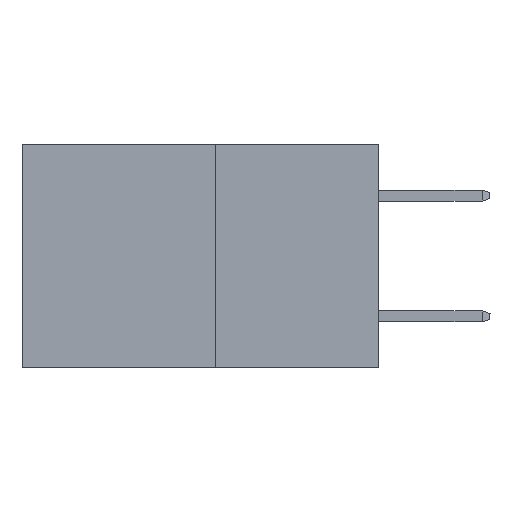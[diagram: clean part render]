
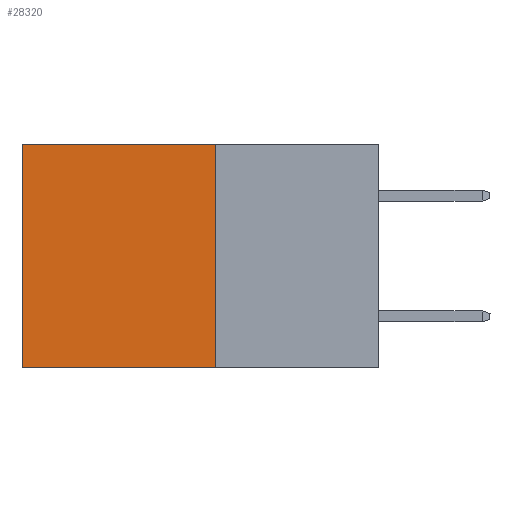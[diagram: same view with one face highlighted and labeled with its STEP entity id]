
A CAD part, left-side view. The second image highlights one B-rep face of the part: STEP entity #28320.
In plain terms, the highlighted planar face has unit normal (-1, 0, 0).
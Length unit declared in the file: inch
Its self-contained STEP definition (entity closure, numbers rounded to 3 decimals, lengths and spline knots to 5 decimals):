
#2869 = EDGE_CURVE ( 'NONE', #17313, #3148, #24031, .T. ) ;
#2882 = CARTESIAN_POINT ( 'NONE',  ( 0.277, 0.59, -0.37 ) ) ;
#3148 = VERTEX_POINT ( 'NONE', #2882 ) ;
#4217 = CARTESIAN_POINT ( 'NONE',  ( 0.277, 0.27, -0.37 ) ) ;
#5641 = ORIENTED_EDGE ( 'NONE', *, *, #2869, .T. ) ;
#6973 = DIRECTION ( 'NONE',  ( 0., 0., -1. ) ) ;
#7343 = LINE ( 'NONE', #17744, #33714 ) ;
#9511 = EDGE_LOOP ( 'NONE', ( #5641, #27579, #11919, #28678 ) ) ;
#10418 = LINE ( 'NONE', #14498, #23711 ) ;
#10582 = CARTESIAN_POINT ( 'NONE',  ( 0.277, 0.27, -0.37 ) ) ;
#11919 = ORIENTED_EDGE ( 'NONE', *, *, #19969, .F. ) ;
#12376 = EDGE_CURVE ( 'NONE', #16581, #17313, #10418, .T. ) ;
#14498 = CARTESIAN_POINT ( 'NONE',  ( 0.277, 0.27, 0. ) ) ;
#16581 = VERTEX_POINT ( 'NONE', #20069 ) ;
#17197 = DIRECTION ( 'NONE',  ( 0., 1., 0. ) ) ;
#17313 = VERTEX_POINT ( 'NONE', #33126 ) ;
#17579 = PLANE ( 'NONE',  #18585 ) ;
#17744 = CARTESIAN_POINT ( 'NONE',  ( 0.277, 0.27, -0.37 ) ) ;
#17836 = VECTOR ( 'NONE', #33476, 39.37008 ) ;
#18463 = VECTOR ( 'NONE', #26418, 39.37008 ) ;
#18585 = AXIS2_PLACEMENT_3D ( 'NONE', #4217, #22906, #6973 ) ;
#19057 = EDGE_CURVE ( 'NONE', #32577, #3148, #7343, .T. ) ;
#19969 = EDGE_CURVE ( 'NONE', #16581, #32577, #25448, .T. ) ;
#20069 = CARTESIAN_POINT ( 'NONE',  ( 0.277, 0.27, 0. ) ) ;
#22906 = DIRECTION ( 'NONE',  ( 1., 0., 0. ) ) ;
#23711 = VECTOR ( 'NONE', #17197, 39.37008 ) ;
#24031 = LINE ( 'NONE', #30747, #17836 ) ;
#24124 = CARTESIAN_POINT ( 'NONE',  ( 0.277, 0.27, -0.37 ) ) ;
#25448 = LINE ( 'NONE', #10582, #18463 ) ;
#26418 = DIRECTION ( 'NONE',  ( 0., 0., -1. ) ) ;
#27579 = ORIENTED_EDGE ( 'NONE', *, *, #19057, .F. ) ;
#28320 = ADVANCED_FACE ( 'NONE', ( #29444 ), #17579, .F. ) ;
#28678 = ORIENTED_EDGE ( 'NONE', *, *, #12376, .T. ) ;
#29444 = FACE_OUTER_BOUND ( 'NONE', #9511, .T. ) ;
#30747 = CARTESIAN_POINT ( 'NONE',  ( 0.277, 0.59, -0.37 ) ) ;
#30752 = DIRECTION ( 'NONE',  ( 0., 1., 0. ) ) ;
#32577 = VERTEX_POINT ( 'NONE', #24124 ) ;
#33126 = CARTESIAN_POINT ( 'NONE',  ( 0.277, 0.59, 0. ) ) ;
#33476 = DIRECTION ( 'NONE',  ( 0., 0., -1. ) ) ;
#33714 = VECTOR ( 'NONE', #30752, 39.37008 ) ;
